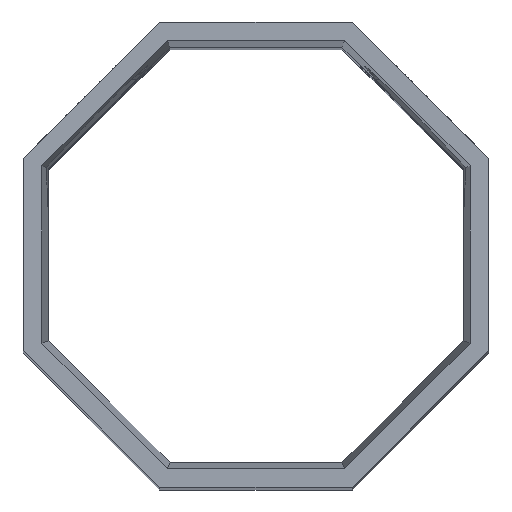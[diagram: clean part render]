
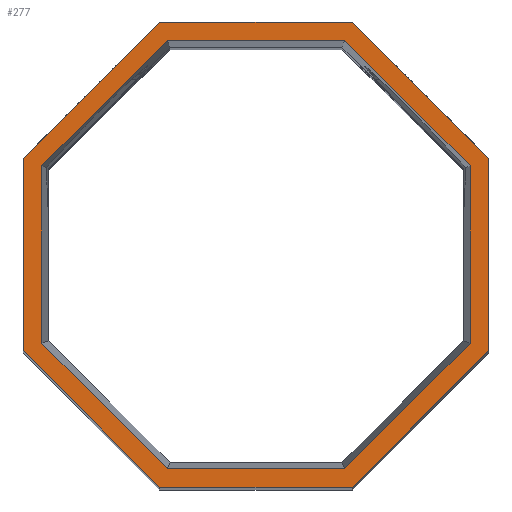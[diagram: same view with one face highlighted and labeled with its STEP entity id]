
A CAD part, top view. The second image highlights one B-rep face of the part: STEP entity #277.
In plain terms, the highlighted planar face has unit normal (0, 0, 1).
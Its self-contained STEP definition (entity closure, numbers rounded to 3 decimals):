
#6 = EDGE_CURVE ( 'NONE', #969, #741, #288, .T. ) ;
#19 = CARTESIAN_POINT ( 'NONE',  ( 2.803, 21.378, 123. ) ) ;
#42 = CARTESIAN_POINT ( 'NONE',  ( -21.378, 2.803, 123. ) ) ;
#54 = VECTOR ( 'NONE', #1056, 1000. ) ;
#72 = EDGE_CURVE ( 'NONE', #606, #2318, #1632, .T. ) ;
#117 = DIRECTION ( 'NONE',  ( 1., 0., 0. ) ) ;
#144 = VECTOR ( 'NONE', #1291, 1000. ) ;
#150 = CARTESIAN_POINT ( 'NONE',  ( 18.575, -7.694, 123. ) ) ;
#241 = CARTESIAN_POINT ( 'NONE',  ( 18.575, -7.694, 123. ) ) ;
#269 = ORIENTED_EDGE ( 'NONE', *, *, #1293, .T. ) ;
#277 = ADVANCED_FACE ( 'NONE', ( #1683, #2682 ), #409, .T. ) ;
#288 = LINE ( 'NONE', #2623, #2492 ) ;
#310 = ORIENTED_EDGE ( 'NONE', *, *, #2211, .T. ) ;
#323 = VECTOR ( 'NONE', #2662, 1000. ) ;
#333 = VECTOR ( 'NONE', #2668, 1000. ) ;
#348 = VERTEX_POINT ( 'NONE', #843 ) ;
#359 = LINE ( 'NONE', #1415, #323 ) ;
#374 = VERTEX_POINT ( 'NONE', #2153 ) ;
#405 = CARTESIAN_POINT ( 'NONE',  ( -18.575, 0., 123. ) ) ;
#409 = PLANE ( 'NONE',  #1742 ) ;
#416 = VECTOR ( 'NONE', #2336, 1000. ) ;
#448 = LINE ( 'NONE', #19, #2604 ) ;
#496 = EDGE_CURVE ( 'NONE', #2730, #2700, #2610, .T. ) ;
#515 = ORIENTED_EDGE ( 'NONE', *, *, #2025, .T. ) ;
#545 = VECTOR ( 'NONE', #556, 1000. ) ;
#556 = DIRECTION ( 'NONE',  ( 0., 1., 0. ) ) ;
#567 = CARTESIAN_POINT ( 'NONE',  ( -18.575, 7.694, 123. ) ) ;
#592 = ORIENTED_EDGE ( 'NONE', *, *, #72, .T. ) ;
#606 = VERTEX_POINT ( 'NONE', #1448 ) ;
#649 = CARTESIAN_POINT ( 'NONE',  ( 2.803, -21.378, 123. ) ) ;
#693 = CARTESIAN_POINT ( 'NONE',  ( 7.694, -18.575, 123. ) ) ;
#708 = VECTOR ( 'NONE', #1543, 1000. ) ;
#728 = DIRECTION ( 'NONE',  ( -0.707, 0.707, 0. ) ) ;
#741 = VERTEX_POINT ( 'NONE', #873 ) ;
#755 = LINE ( 'NONE', #2198, #333 ) ;
#763 = VERTEX_POINT ( 'NONE', #1540 ) ;
#784 = CARTESIAN_POINT ( 'NONE',  ( -18.575, 0., 123. ) ) ;
#806 = ORIENTED_EDGE ( 'NONE', *, *, #2284, .T. ) ;
#824 = DIRECTION ( 'NONE',  ( 0., -1., 0. ) ) ;
#825 = LINE ( 'NONE', #1904, #54 ) ;
#833 = ORIENTED_EDGE ( 'NONE', *, *, #2582, .T. ) ;
#843 = CARTESIAN_POINT ( 'NONE',  ( -7.083, 17.099, 123. ) ) ;
#852 = CARTESIAN_POINT ( 'NONE',  ( -21.378, -2.803, 123. ) ) ;
#868 = CARTESIAN_POINT ( 'NONE',  ( 7.083, -17.099, 123. ) ) ;
#871 = ORIENTED_EDGE ( 'NONE', *, *, #2335, .T. ) ;
#873 = CARTESIAN_POINT ( 'NONE',  ( -7.694, -18.575, 123. ) ) ;
#888 = EDGE_LOOP ( 'NONE', ( #1866, #806, #833, #1824, #310, #2079, #592, #948 ) ) ;
#919 = ORIENTED_EDGE ( 'NONE', *, *, #1890, .T. ) ;
#944 = VECTOR ( 'NONE', #117, 1000. ) ;
#948 = ORIENTED_EDGE ( 'NONE', *, *, #2258, .T. ) ;
#969 = VERTEX_POINT ( 'NONE', #1204 ) ;
#974 = DIRECTION ( 'NONE',  ( 0., 0., 1. ) ) ;
#986 = LINE ( 'NONE', #150, #2476 ) ;
#997 = ORIENTED_EDGE ( 'NONE', *, *, #6, .T. ) ;
#1053 = VECTOR ( 'NONE', #2669, 1000. ) ;
#1056 = DIRECTION ( 'NONE',  ( -1., 0., 0. ) ) ;
#1062 = DIRECTION ( 'NONE',  ( 0.707, -0.707, 0. ) ) ;
#1070 = CARTESIAN_POINT ( 'NONE',  ( 17.099, -7.083, 123. ) ) ;
#1098 = EDGE_LOOP ( 'NONE', ( #2313, #871, #997, #269, #1316, #919, #1613, #515 ) ) ;
#1123 = VECTOR ( 'NONE', #728, 1000. ) ;
#1204 = CARTESIAN_POINT ( 'NONE',  ( -18.575, -7.694, 123. ) ) ;
#1235 = LINE ( 'NONE', #405, #2516 ) ;
#1249 = LINE ( 'NONE', #649, #416 ) ;
#1291 = DIRECTION ( 'NONE',  ( -0.707, 0.707, 0. ) ) ;
#1293 = EDGE_CURVE ( 'NONE', #741, #2730, #1827, .T. ) ;
#1316 = ORIENTED_EDGE ( 'NONE', *, *, #496, .T. ) ;
#1406 = VERTEX_POINT ( 'NONE', #1640 ) ;
#1415 = CARTESIAN_POINT ( 'NONE',  ( -7.694, 18.575, 123. ) ) ;
#1448 = CARTESIAN_POINT ( 'NONE',  ( 17.099, 7.083, 123. ) ) ;
#1483 = CARTESIAN_POINT ( 'NONE',  ( 7.694, -18.575, 123. ) ) ;
#1487 = VERTEX_POINT ( 'NONE', #567 ) ;
#1540 = CARTESIAN_POINT ( 'NONE',  ( 7.694, 18.575, 123. ) ) ;
#1542 = DIRECTION ( 'NONE',  ( 0.707, -0.707, 0. ) ) ;
#1543 = DIRECTION ( 'NONE',  ( 0.707, 0.707, 0. ) ) ;
#1573 = VECTOR ( 'NONE', #1727, 1000. ) ;
#1609 = CARTESIAN_POINT ( 'NONE',  ( -7.694, -18.575, 123. ) ) ;
#1613 = ORIENTED_EDGE ( 'NONE', *, *, #2081, .T. ) ;
#1622 = DIRECTION ( 'NONE',  ( 0., -1., 0. ) ) ;
#1632 = LINE ( 'NONE', #2293, #2007 ) ;
#1640 = CARTESIAN_POINT ( 'NONE',  ( -7.083, -17.099, 123. ) ) ;
#1683 = FACE_BOUND ( 'NONE', #888, .T. ) ;
#1727 = DIRECTION ( 'NONE',  ( 0.707, 0.707, 0. ) ) ;
#1742 = AXIS2_PLACEMENT_3D ( 'NONE', #784, #974, #1622 ) ;
#1796 = LINE ( 'NONE', #2640, #1123 ) ;
#1824 = ORIENTED_EDGE ( 'NONE', *, *, #2705, .T. ) ;
#1827 = LINE ( 'NONE', #1609, #1053 ) ;
#1866 = ORIENTED_EDGE ( 'NONE', *, *, #2375, .T. ) ;
#1872 = VERTEX_POINT ( 'NONE', #2116 ) ;
#1890 = EDGE_CURVE ( 'NONE', #2700, #374, #986, .T. ) ;
#1904 = CARTESIAN_POINT ( 'NONE',  ( -18.575, -17.099, 123. ) ) ;
#1933 = DIRECTION ( 'NONE',  ( 0., -1., 0. ) ) ;
#2007 = VECTOR ( 'NONE', #824, 1000. ) ;
#2025 = EDGE_CURVE ( 'NONE', #763, #2374, #755, .T. ) ;
#2060 = DIRECTION ( 'NONE',  ( 0., 1., 0. ) ) ;
#2079 = ORIENTED_EDGE ( 'NONE', *, *, #2635, .T. ) ;
#2081 = EDGE_CURVE ( 'NONE', #374, #763, #1796, .T. ) ;
#2113 = LINE ( 'NONE', #852, #144 ) ;
#2116 = CARTESIAN_POINT ( 'NONE',  ( 7.083, 17.099, 123. ) ) ;
#2140 = CARTESIAN_POINT ( 'NONE',  ( -7.694, 18.575, 123. ) ) ;
#2151 = CARTESIAN_POINT ( 'NONE',  ( -17.099, -7.083, 123. ) ) ;
#2153 = CARTESIAN_POINT ( 'NONE',  ( 18.575, 7.694, 123. ) ) ;
#2192 = EDGE_CURVE ( 'NONE', #2374, #1487, #359, .T. ) ;
#2198 = CARTESIAN_POINT ( 'NONE',  ( 7.694, 18.575, 123. ) ) ;
#2211 = EDGE_CURVE ( 'NONE', #348, #1872, #2250, .T. ) ;
#2250 = LINE ( 'NONE', #2708, #944 ) ;
#2258 = EDGE_CURVE ( 'NONE', #2318, #2684, #1249, .T. ) ;
#2280 = VERTEX_POINT ( 'NONE', #2151 ) ;
#2284 = EDGE_CURVE ( 'NONE', #1406, #2280, #2113, .T. ) ;
#2293 = CARTESIAN_POINT ( 'NONE',  ( 17.099, 0., 123. ) ) ;
#2313 = ORIENTED_EDGE ( 'NONE', *, *, #2192, .T. ) ;
#2318 = VERTEX_POINT ( 'NONE', #1070 ) ;
#2335 = EDGE_CURVE ( 'NONE', #1487, #969, #1235, .T. ) ;
#2336 = DIRECTION ( 'NONE',  ( -0.707, -0.707, 0. ) ) ;
#2355 = LINE ( 'NONE', #42, #1573 ) ;
#2374 = VERTEX_POINT ( 'NONE', #2140 ) ;
#2375 = EDGE_CURVE ( 'NONE', #2684, #1406, #825, .T. ) ;
#2475 = CARTESIAN_POINT ( 'NONE',  ( -17.099, 0., 123. ) ) ;
#2476 = VECTOR ( 'NONE', #2060, 1000. ) ;
#2492 = VECTOR ( 'NONE', #1542, 1000. ) ;
#2516 = VECTOR ( 'NONE', #1933, 1000. ) ;
#2553 = CARTESIAN_POINT ( 'NONE',  ( -17.099, 7.083, 123. ) ) ;
#2582 = EDGE_CURVE ( 'NONE', #2280, #2677, #2701, .T. ) ;
#2604 = VECTOR ( 'NONE', #1062, 1000. ) ;
#2610 = LINE ( 'NONE', #693, #708 ) ;
#2623 = CARTESIAN_POINT ( 'NONE',  ( -18.575, -7.694, 123. ) ) ;
#2635 = EDGE_CURVE ( 'NONE', #1872, #606, #448, .T. ) ;
#2640 = CARTESIAN_POINT ( 'NONE',  ( 18.575, 7.694, 123. ) ) ;
#2662 = DIRECTION ( 'NONE',  ( -0.707, -0.707, 0. ) ) ;
#2668 = DIRECTION ( 'NONE',  ( -1., 0., 0. ) ) ;
#2669 = DIRECTION ( 'NONE',  ( 1., 0., 0. ) ) ;
#2677 = VERTEX_POINT ( 'NONE', #2553 ) ;
#2682 = FACE_OUTER_BOUND ( 'NONE', #1098, .T. ) ;
#2684 = VERTEX_POINT ( 'NONE', #868 ) ;
#2700 = VERTEX_POINT ( 'NONE', #241 ) ;
#2701 = LINE ( 'NONE', #2475, #545 ) ;
#2705 = EDGE_CURVE ( 'NONE', #2677, #348, #2355, .T. ) ;
#2708 = CARTESIAN_POINT ( 'NONE',  ( -18.575, 17.099, 123. ) ) ;
#2730 = VERTEX_POINT ( 'NONE', #1483 ) ;
